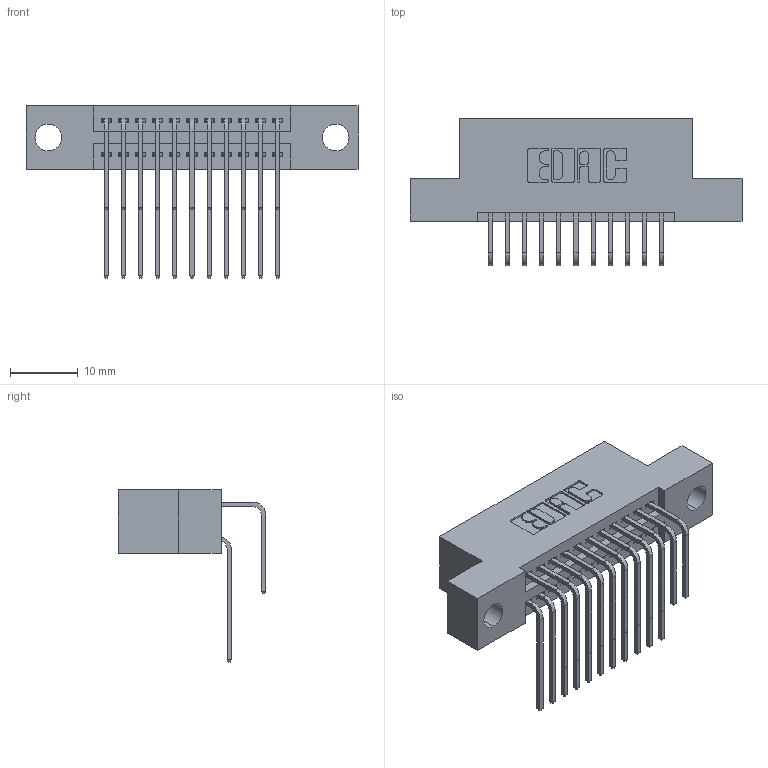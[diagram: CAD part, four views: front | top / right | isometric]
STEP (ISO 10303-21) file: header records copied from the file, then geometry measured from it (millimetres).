
FILE_DESCRIPTION (( 'STEP AP203' ), '1' );
FILE_NAME ('345-022-558-204.STEP', '2018-08-21T00:50:25', ( '' ), ( '' ), 'SwSTEP 2.0', 'SolidWorks 2016', '' );
FILE_SCHEMA (( 'CONFIG_CONTROL_DESIGN' ));
Length unit declared in the file: inch
Products named in the file (4): 345-292-001_558 559 Tail - 1; 345-292-001_558 Tail - 2; 345-022-558-204; 345 Part_Flush Mounting Lugs - 0.156 Dia-TH
Assembly tree (23 placements, depth 2):
  345-022-558-204
    345 Part_Flush Mounting Lugs - 0.156 Dia-TH
    345-292-001_558 559 Tail - 1  x11
    345-292-001_558 Tail - 2  x11
Bounding box: 49.15 x 21.83 x 25.53 mm (x, y, z)
Volume: 4525.7 mm3; surface area: 6501.3 mm2
Topology: 23 solids, 23 shells, 1270 faces, 3751 edges, 2470 vertices
Faces by surface type: plane 850, cylinder 420
Entity records: 14459 total; most frequent: CARTESIAN_POINT 2499, ORIENTED_EDGE 2382, DIRECTION 2215, EDGE_CURVE 1191, LINE 975, VECTOR 975, VERTEX_POINT 790, AXIS2_PLACEMENT_3D 620
